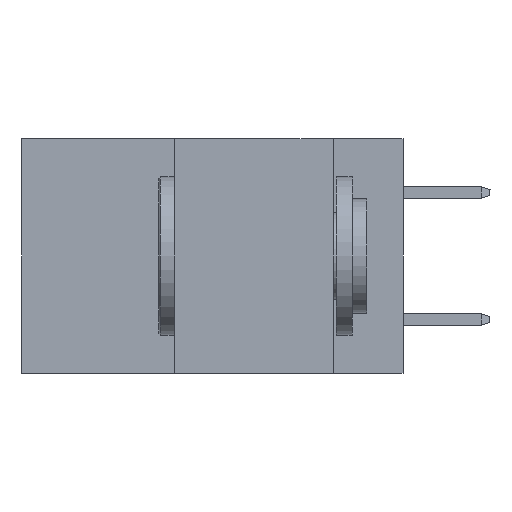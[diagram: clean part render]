
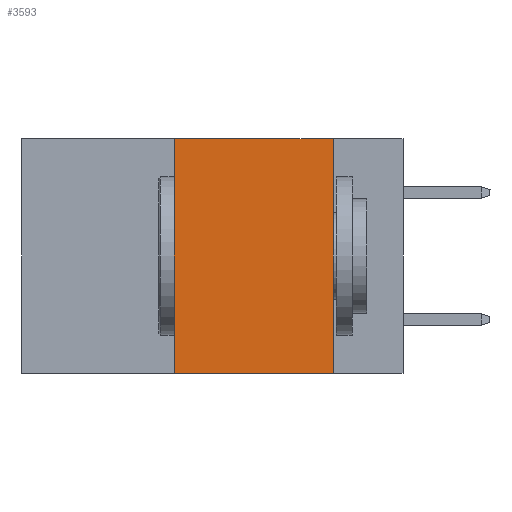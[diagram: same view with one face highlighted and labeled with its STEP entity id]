
A CAD part, left-side view. The second image highlights one B-rep face of the part: STEP entity #3593.
In plain terms, the highlighted planar face has unit normal (-1, 0, 0).
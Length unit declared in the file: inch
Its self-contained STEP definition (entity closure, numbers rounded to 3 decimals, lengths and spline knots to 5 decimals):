
#36 = EDGE_CURVE ( 'NONE', #1715, #22242, #10571, .T. ) ;
#677 = ORIENTED_EDGE ( 'NONE', *, *, #36, .F. ) ;
#758 = CARTESIAN_POINT ( 'NONE',  ( 0., 0.36, 0. ) ) ;
#1715 = VERTEX_POINT ( 'NONE', #42016 ) ;
#3593 = ADVANCED_FACE ( 'NONE', ( #11499 ), #31655, .F. ) ;
#3888 = DIRECTION ( 'NONE',  ( 0., -1., 0. ) ) ;
#4049 = CARTESIAN_POINT ( 'NONE',  ( 0., 0.36, 0. ) ) ;
#4623 = CARTESIAN_POINT ( 'NONE',  ( 0., 0.11, -0.37 ) ) ;
#6100 = VECTOR ( 'NONE', #3888, 39.37008 ) ;
#6577 = CARTESIAN_POINT ( 'NONE',  ( 0., 0.11, 0. ) ) ;
#7712 = AXIS2_PLACEMENT_3D ( 'NONE', #18193, #22240, #8814 ) ;
#8749 = VECTOR ( 'NONE', #36621, 39.37008 ) ;
#8814 = DIRECTION ( 'NONE',  ( 0., 0., -1. ) ) ;
#9030 = EDGE_CURVE ( 'NONE', #21452, #13653, #9965, .T. ) ;
#9965 = LINE ( 'NONE', #6577, #8749 ) ;
#10571 = LINE ( 'NONE', #4049, #37424 ) ;
#11184 = ORIENTED_EDGE ( 'NONE', *, *, #12065, .F. ) ;
#11444 = EDGE_CURVE ( 'NONE', #1715, #13653, #12574, .T. ) ;
#11499 = FACE_OUTER_BOUND ( 'NONE', #36390, .T. ) ;
#12065 = EDGE_CURVE ( 'NONE', #22242, #21452, #13978, .T. ) ;
#12574 = LINE ( 'NONE', #26226, #13240 ) ;
#13240 = VECTOR ( 'NONE', #25563, 39.37008 ) ;
#13653 = VERTEX_POINT ( 'NONE', #4623 ) ;
#13978 = LINE ( 'NONE', #34587, #6100 ) ;
#18193 = CARTESIAN_POINT ( 'NONE',  ( 0., 0.6, 0. ) ) ;
#21452 = VERTEX_POINT ( 'NONE', #23458 ) ;
#22240 = DIRECTION ( 'NONE',  ( 1., 0., 0. ) ) ;
#22242 = VERTEX_POINT ( 'NONE', #758 ) ;
#23458 = CARTESIAN_POINT ( 'NONE',  ( 0., 0.11, 0. ) ) ;
#25563 = DIRECTION ( 'NONE',  ( 0., -1., 0. ) ) ;
#26226 = CARTESIAN_POINT ( 'NONE',  ( 0., 0.6, -0.37 ) ) ;
#29708 = ORIENTED_EDGE ( 'NONE', *, *, #9030, .F. ) ;
#31655 = PLANE ( 'NONE',  #7712 ) ;
#34587 = CARTESIAN_POINT ( 'NONE',  ( 0., 0.6, 0. ) ) ;
#36390 = EDGE_LOOP ( 'NONE', ( #29708, #11184, #677, #39810 ) ) ;
#36621 = DIRECTION ( 'NONE',  ( 0., 0., -1. ) ) ;
#37424 = VECTOR ( 'NONE', #38323, 39.37008 ) ;
#38323 = DIRECTION ( 'NONE',  ( 0., 0., 1. ) ) ;
#39810 = ORIENTED_EDGE ( 'NONE', *, *, #11444, .T. ) ;
#42016 = CARTESIAN_POINT ( 'NONE',  ( 0., 0.36, -0.37 ) ) ;
